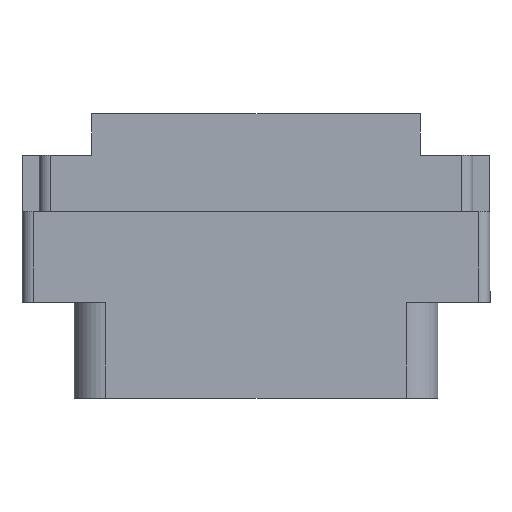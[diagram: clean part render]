
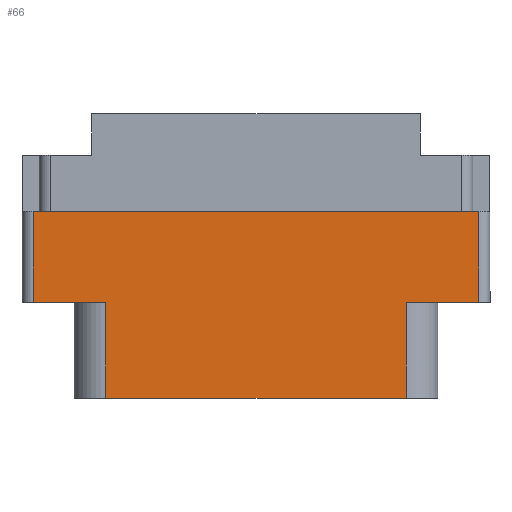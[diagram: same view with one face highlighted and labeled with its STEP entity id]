
A CAD part, front view. The second image highlights one B-rep face of the part: STEP entity #66.
In plain terms, the highlighted planar face has unit normal (0, -1, 0).
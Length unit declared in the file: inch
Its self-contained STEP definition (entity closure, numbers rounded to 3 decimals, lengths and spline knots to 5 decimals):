
#66 = ADVANCED_FACE ( 'NONE', ( #16583 ), #12433, .T. ) ;
#231 = EDGE_CURVE ( 'NONE', #23097, #11576, #6321, .T. ) ;
#441 = EDGE_CURVE ( 'NONE', #11576, #8274, #22919, .T. ) ;
#1096 = CARTESIAN_POINT ( 'NONE',  ( 0., -0.343, -0.529 ) ) ;
#2425 = CARTESIAN_POINT ( 'NONE',  ( 0.624, -0.343, -0.798 ) ) ;
#3469 = CARTESIAN_POINT ( 'NONE',  ( -0.42052, -0.343, -0.798 ) ) ;
#3619 = VERTEX_POINT ( 'NONE', #24861 ) ;
#4925 = CARTESIAN_POINT ( 'NONE',  ( -0.624, -0.343, -0.798 ) ) ;
#5709 = ORIENTED_EDGE ( 'NONE', *, *, #10955, .F. ) ;
#6271 = LINE ( 'NONE', #12318, #18334 ) ;
#6321 = LINE ( 'NONE', #22773, #21089 ) ;
#6370 = DIRECTION ( 'NONE',  ( 0., 0., 1. ) ) ;
#6875 = DIRECTION ( 'NONE',  ( 0., 0., -1. ) ) ;
#6895 = DIRECTION ( 'NONE',  ( 0., 0., 1. ) ) ;
#7754 = LINE ( 'NONE', #1096, #11647 ) ;
#8167 = ORIENTED_EDGE ( 'NONE', *, *, #10125, .F. ) ;
#8274 = VERTEX_POINT ( 'NONE', #11016 ) ;
#8310 = DIRECTION ( 'NONE',  ( 1., 0., 0. ) ) ;
#8510 = VERTEX_POINT ( 'NONE', #23591 ) ;
#8655 = AXIS2_PLACEMENT_3D ( 'NONE', #21824, #20141, #23783 ) ;
#8740 = CARTESIAN_POINT ( 'NONE',  ( -0.624, -0.343, -0.274 ) ) ;
#9459 = EDGE_CURVE ( 'NONE', #13177, #8510, #25017, .T. ) ;
#9761 = CARTESIAN_POINT ( 'NONE',  ( 0., -0.343, -0.529 ) ) ;
#10125 = EDGE_CURVE ( 'NONE', #12041, #17787, #6271, .T. ) ;
#10190 = CARTESIAN_POINT ( 'NONE',  ( -0.624, -0.343, -0.529 ) ) ;
#10955 = EDGE_CURVE ( 'NONE', #3619, #8274, #7754, .T. ) ;
#10958 = ORIENTED_EDGE ( 'NONE', *, *, #9459, .T. ) ;
#11016 = CARTESIAN_POINT ( 'NONE',  ( 0.42052, -0.343, -0.529 ) ) ;
#11576 = VERTEX_POINT ( 'NONE', #22469 ) ;
#11647 = VECTOR ( 'NONE', #24132, 39.37008 ) ;
#11655 = ORIENTED_EDGE ( 'NONE', *, *, #23357, .T. ) ;
#12041 = VERTEX_POINT ( 'NONE', #8740 ) ;
#12142 = LINE ( 'NONE', #2425, #21818 ) ;
#12318 = CARTESIAN_POINT ( 'NONE',  ( 0., -0.343, -0.274 ) ) ;
#12393 = EDGE_LOOP ( 'NONE', ( #8167, #15419, #10958, #14379, #15181, #19045, #5709, #11655 ) ) ;
#12433 = PLANE ( 'NONE',  #8655 ) ;
#12657 = EDGE_CURVE ( 'NONE', #8510, #23097, #18558, .T. ) ;
#13177 = VERTEX_POINT ( 'NONE', #10190 ) ;
#13715 = VECTOR ( 'NONE', #22176, 39.37008 ) ;
#14379 = ORIENTED_EDGE ( 'NONE', *, *, #12657, .T. ) ;
#14699 = CARTESIAN_POINT ( 'NONE',  ( 0.42052, -0.343, -0.529 ) ) ;
#15181 = ORIENTED_EDGE ( 'NONE', *, *, #231, .T. ) ;
#15419 = ORIENTED_EDGE ( 'NONE', *, *, #22207, .T. ) ;
#15649 = VECTOR ( 'NONE', #6895, 39.37008 ) ;
#16482 = CARTESIAN_POINT ( 'NONE',  ( -0.42052, -0.343, -0.798 ) ) ;
#16583 = FACE_OUTER_BOUND ( 'NONE', #12393, .T. ) ;
#17258 = CARTESIAN_POINT ( 'NONE',  ( 0.624, -0.343, -0.274 ) ) ;
#17599 = DIRECTION ( 'NONE',  ( 1., 0., 0. ) ) ;
#17787 = VERTEX_POINT ( 'NONE', #17258 ) ;
#18334 = VECTOR ( 'NONE', #8310, 39.37008 ) ;
#18558 = LINE ( 'NONE', #16482, #24625 ) ;
#19045 = ORIENTED_EDGE ( 'NONE', *, *, #441, .T. ) ;
#19281 = VECTOR ( 'NONE', #21729, 39.37008 ) ;
#20141 = DIRECTION ( 'NONE',  ( 0., -1., 0. ) ) ;
#21089 = VECTOR ( 'NONE', #17599, 39.37008 ) ;
#21729 = DIRECTION ( 'NONE',  ( 1., 0., 0. ) ) ;
#21818 = VECTOR ( 'NONE', #6370, 39.37008 ) ;
#21824 = CARTESIAN_POINT ( 'NONE',  ( -0.656, -0.343, -0.798 ) ) ;
#22176 = DIRECTION ( 'NONE',  ( 0., 0., -1. ) ) ;
#22178 = LINE ( 'NONE', #4925, #13715 ) ;
#22207 = EDGE_CURVE ( 'NONE', #12041, #13177, #22178, .T. ) ;
#22469 = CARTESIAN_POINT ( 'NONE',  ( 0.42052, -0.343, -0.798 ) ) ;
#22773 = CARTESIAN_POINT ( 'NONE',  ( -0.656, -0.343, -0.798 ) ) ;
#22919 = LINE ( 'NONE', #14699, #15649 ) ;
#23097 = VERTEX_POINT ( 'NONE', #3469 ) ;
#23357 = EDGE_CURVE ( 'NONE', #3619, #17787, #12142, .T. ) ;
#23591 = CARTESIAN_POINT ( 'NONE',  ( -0.42052, -0.343, -0.529 ) ) ;
#23783 = DIRECTION ( 'NONE',  ( 0., 0., -1. ) ) ;
#24132 = DIRECTION ( 'NONE',  ( -1., 0., 0. ) ) ;
#24625 = VECTOR ( 'NONE', #6875, 39.37008 ) ;
#24861 = CARTESIAN_POINT ( 'NONE',  ( 0.624, -0.343, -0.529 ) ) ;
#25017 = LINE ( 'NONE', #9761, #19281 ) ;
